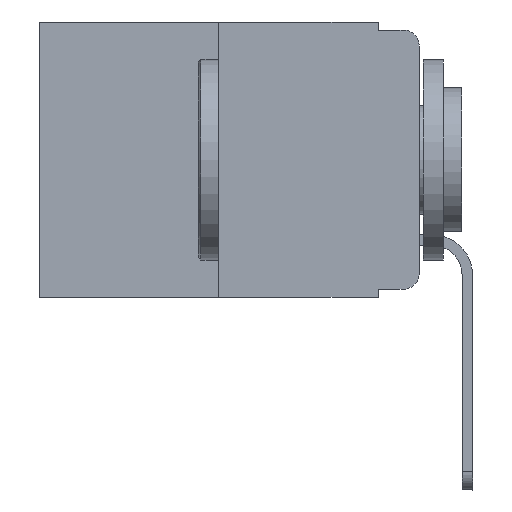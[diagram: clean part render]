
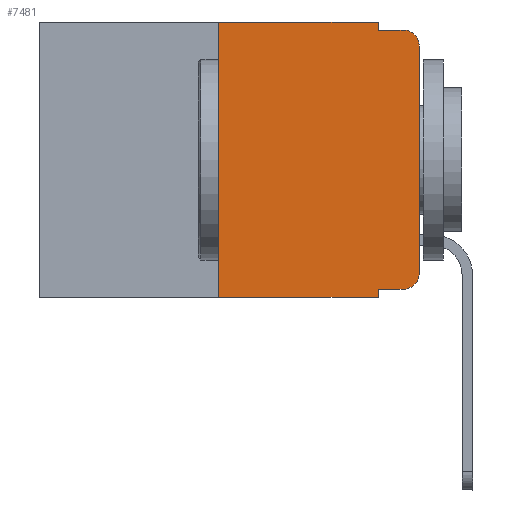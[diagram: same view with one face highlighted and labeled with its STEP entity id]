
A CAD part, left-side view. The second image highlights one B-rep face of the part: STEP entity #7481.
In plain terms, the highlighted planar face has unit normal (-1, 0, 0).
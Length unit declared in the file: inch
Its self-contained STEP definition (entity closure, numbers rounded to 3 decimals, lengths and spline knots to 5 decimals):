
#312 = FACE_OUTER_BOUND ( 'NONE', #12741, .T. ) ;
#485 = DIRECTION ( 'NONE',  ( 0., 0., 1. ) ) ;
#605 = ORIENTED_EDGE ( 'NONE', *, *, #1512, .T. ) ;
#611 = VERTEX_POINT ( 'NONE', #9540 ) ;
#612 = CIRCLE ( 'NONE', #8128, 0.02 ) ;
#677 = VERTEX_POINT ( 'NONE', #10456 ) ;
#765 = VERTEX_POINT ( 'NONE', #8764 ) ;
#1247 = VECTOR ( 'NONE', #1843, 39.37008 ) ;
#1512 = EDGE_CURVE ( 'NONE', #2712, #677, #11167, .T. ) ;
#1531 = EDGE_CURVE ( 'NONE', #677, #3654, #7296, .T. ) ;
#1843 = DIRECTION ( 'NONE',  ( 0., -1., 0. ) ) ;
#1937 = DIRECTION ( 'NONE',  ( 0., 0., -1. ) ) ;
#2383 = DIRECTION ( 'NONE',  ( 1., 0., 0. ) ) ;
#2686 = CARTESIAN_POINT ( 'NONE',  ( 0., 0., -0.03 ) ) ;
#2712 = VERTEX_POINT ( 'NONE', #6951 ) ;
#2860 = VERTEX_POINT ( 'NONE', #6246 ) ;
#3067 = CARTESIAN_POINT ( 'NONE',  ( 0., 0., 0. ) ) ;
#3071 = CARTESIAN_POINT ( 'NONE',  ( 0., 0.051, -0.343 ) ) ;
#3164 = DIRECTION ( 'NONE',  ( 0., 0., -1. ) ) ;
#3264 = ORIENTED_EDGE ( 'NONE', *, *, #4771, .F. ) ;
#3280 = VERTEX_POINT ( 'NONE', #6628 ) ;
#3393 = ORIENTED_EDGE ( 'NONE', *, *, #1531, .T. ) ;
#3524 = VECTOR ( 'NONE', #11157, 39.37008 ) ;
#3654 = VERTEX_POINT ( 'NONE', #2686 ) ;
#3736 = EDGE_CURVE ( 'NONE', #10041, #611, #7381, .T. ) ;
#3966 = DIRECTION ( 'NONE',  ( 0., 0., -1. ) ) ;
#4029 = DIRECTION ( 'NONE',  ( 0., 0., -1. ) ) ;
#4185 = VERTEX_POINT ( 'NONE', #3071 ) ;
#4205 = EDGE_CURVE ( 'NONE', #10310, #4185, #11339, .T. ) ;
#4398 = VECTOR ( 'NONE', #12665, 39.37008 ) ;
#4546 = DIRECTION ( 'NONE',  ( 0., -1., 0. ) ) ;
#4619 = CARTESIAN_POINT ( 'NONE',  ( 0., 0.473, 0. ) ) ;
#4771 = EDGE_CURVE ( 'NONE', #10310, #10041, #6574, .T. ) ;
#4973 = CARTESIAN_POINT ( 'NONE',  ( 0., 0.051, 0. ) ) ;
#5005 = DIRECTION ( 'NONE',  ( -1., 0., 0. ) ) ;
#5068 = LINE ( 'NONE', #9309, #7281 ) ;
#6044 = CARTESIAN_POINT ( 'NONE',  ( 0., 0.02, -0.313 ) ) ;
#6246 = CARTESIAN_POINT ( 'NONE',  ( 0., 0.051, -0.333 ) ) ;
#6532 = ORIENTED_EDGE ( 'NONE', *, *, #4205, .T. ) ;
#6574 = LINE ( 'NONE', #10885, #8964 ) ;
#6628 = CARTESIAN_POINT ( 'NONE',  ( 0., 0.02, -0.01 ) ) ;
#6694 = EDGE_CURVE ( 'NONE', #3654, #3280, #612, .T. ) ;
#6951 = CARTESIAN_POINT ( 'NONE',  ( 0., 0.02, -0.333 ) ) ;
#7253 = LINE ( 'NONE', #4973, #11330 ) ;
#7281 = VECTOR ( 'NONE', #4029, 39.37008 ) ;
#7296 = LINE ( 'NONE', #3067, #10727 ) ;
#7303 = CARTESIAN_POINT ( 'NONE',  ( 0., 0.473, -0.343 ) ) ;
#7381 = LINE ( 'NONE', #8414, #4398 ) ;
#7481 = ADVANCED_FACE ( 'NONE', ( #312 ), #11897, .F. ) ;
#7872 = ORIENTED_EDGE ( 'NONE', *, *, #8205, .F. ) ;
#8128 = AXIS2_PLACEMENT_3D ( 'NONE', #9534, #10514, #3164 ) ;
#8205 = EDGE_CURVE ( 'NONE', #611, #765, #5068, .T. ) ;
#8414 = CARTESIAN_POINT ( 'NONE',  ( 0., 0.473, 0. ) ) ;
#8426 = ORIENTED_EDGE ( 'NONE', *, *, #3736, .F. ) ;
#8764 = CARTESIAN_POINT ( 'NONE',  ( 0., 0.051, -0.01 ) ) ;
#8783 = LINE ( 'NONE', #9560, #3524 ) ;
#8825 = DIRECTION ( 'NONE',  ( 0., 0., -1. ) ) ;
#8901 = ORIENTED_EDGE ( 'NONE', *, *, #12270, .T. ) ;
#8938 = ORIENTED_EDGE ( 'NONE', *, *, #11957, .F. ) ;
#8964 = VECTOR ( 'NONE', #485, 39.37008 ) ;
#9264 = AXIS2_PLACEMENT_3D ( 'NONE', #4619, #2383, #8825 ) ;
#9309 = CARTESIAN_POINT ( 'NONE',  ( 0., 0.051, 0. ) ) ;
#9534 = CARTESIAN_POINT ( 'NONE',  ( 0., 0.02, -0.03 ) ) ;
#9540 = CARTESIAN_POINT ( 'NONE',  ( 0., 0.051, 0. ) ) ;
#9560 = CARTESIAN_POINT ( 'NONE',  ( 0., 0.051, -0.01 ) ) ;
#10017 = CARTESIAN_POINT ( 'NONE',  ( 0., 0.051, -0.333 ) ) ;
#10041 = VERTEX_POINT ( 'NONE', #12889 ) ;
#10081 = EDGE_CURVE ( 'NONE', #765, #3280, #8783, .T. ) ;
#10310 = VERTEX_POINT ( 'NONE', #12675 ) ;
#10456 = CARTESIAN_POINT ( 'NONE',  ( 0., 0., -0.313 ) ) ;
#10514 = DIRECTION ( 'NONE',  ( -1., 0., 0. ) ) ;
#10727 = VECTOR ( 'NONE', #11542, 39.37008 ) ;
#10885 = CARTESIAN_POINT ( 'NONE',  ( 0., 0.25, 0. ) ) ;
#11157 = DIRECTION ( 'NONE',  ( 0., -1., 0. ) ) ;
#11167 = CIRCLE ( 'NONE', #12719, 0.02 ) ;
#11330 = VECTOR ( 'NONE', #1937, 39.37008 ) ;
#11339 = LINE ( 'NONE', #7303, #1247 ) ;
#11542 = DIRECTION ( 'NONE',  ( 0., 0., 1. ) ) ;
#11584 = ORIENTED_EDGE ( 'NONE', *, *, #10081, .F. ) ;
#11897 = PLANE ( 'NONE',  #9264 ) ;
#11957 = EDGE_CURVE ( 'NONE', #2860, #4185, #7253, .T. ) ;
#12270 = EDGE_CURVE ( 'NONE', #2860, #2712, #13000, .T. ) ;
#12665 = DIRECTION ( 'NONE',  ( 0., -1., 0. ) ) ;
#12675 = CARTESIAN_POINT ( 'NONE',  ( 0., 0.25, -0.343 ) ) ;
#12719 = AXIS2_PLACEMENT_3D ( 'NONE', #6044, #5005, #3966 ) ;
#12741 = EDGE_LOOP ( 'NONE', ( #3393, #12774, #11584, #7872, #8426, #3264, #6532, #8938, #8901, #605 ) ) ;
#12774 = ORIENTED_EDGE ( 'NONE', *, *, #6694, .T. ) ;
#12889 = CARTESIAN_POINT ( 'NONE',  ( 0., 0.25, 0. ) ) ;
#13000 = LINE ( 'NONE', #10017, #13092 ) ;
#13092 = VECTOR ( 'NONE', #4546, 39.37008 ) ;
